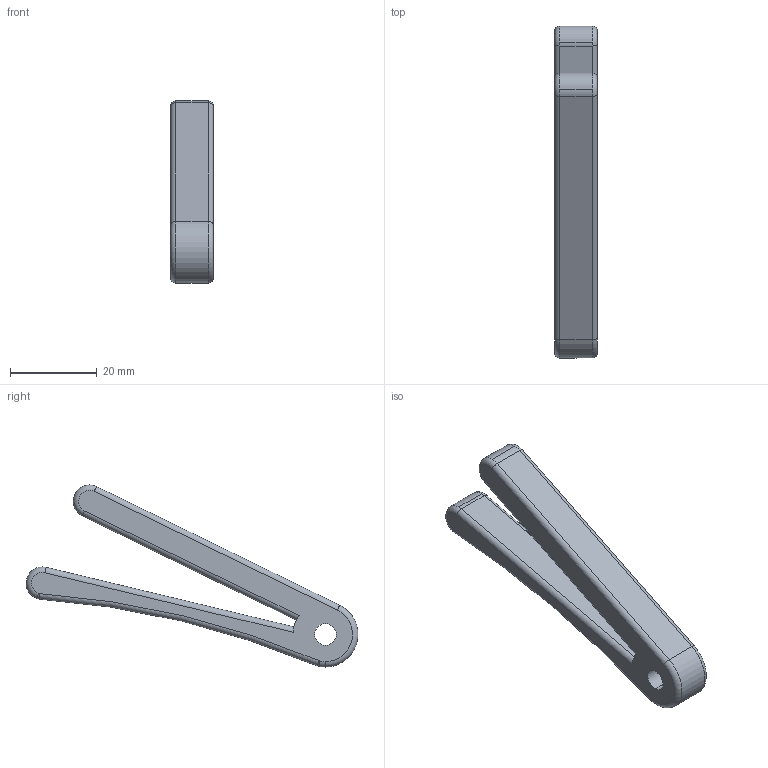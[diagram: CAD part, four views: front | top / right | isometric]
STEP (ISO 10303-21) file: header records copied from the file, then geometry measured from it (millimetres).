
FILE_DESCRIPTION (( 'STEP AP214' ), '1' );
FILE_NAME ('Main_Spring.STEP', '2014-02-20T01:38:06', ( '' ), ( '' ), 'SwSTEP 2.0', 'SolidWorks 2013', '' );
FILE_SCHEMA (( 'AUTOMOTIVE_DESIGN' ));
Length unit declared in the file: millimetre
Products named in the file (1): Main_Spring
Bounding box: 9.9 x 76.53 x 41.97 mm (x, y, z)
Volume: 9266.5 mm3; surface area: 4624.3 mm2
Topology: 1 solids, 1 shells, 36 faces, 86 edges, 52 vertices
Faces by surface type: cylinder 17, torus 14, plane 5
Entity records: 1132 total; most frequent: CARTESIAN_POINT 219, DIRECTION 212, ORIENTED_EDGE 172, AXIS2_PLACEMENT_3D 93, EDGE_CURVE 86, CIRCLE 56, VERTEX_POINT 52, EDGE_LOOP 38
